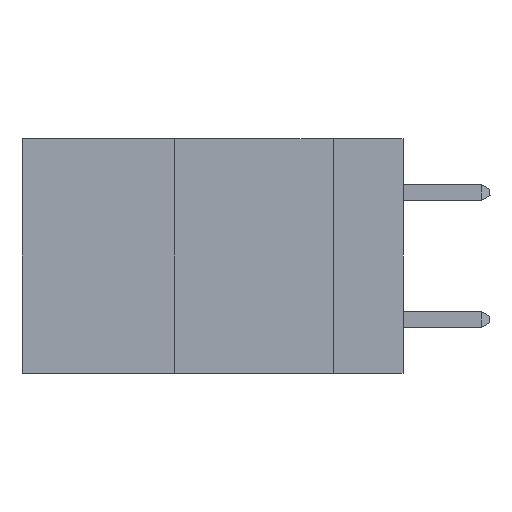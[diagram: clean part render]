
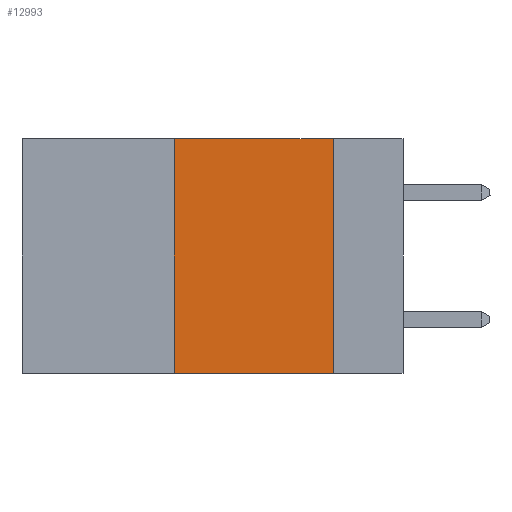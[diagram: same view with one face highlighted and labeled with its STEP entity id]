
A CAD part, left-side view. The second image highlights one B-rep face of the part: STEP entity #12993.
In plain terms, the highlighted planar face has unit normal (-1, 0, 0).
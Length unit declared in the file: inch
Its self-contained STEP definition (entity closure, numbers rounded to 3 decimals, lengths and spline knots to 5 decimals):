
#25 = CARTESIAN_POINT ( 'NONE',  ( 0., 0.36, 0. ) ) ;
#50 = CARTESIAN_POINT ( 'NONE',  ( 0., 0.6, 0. ) ) ;
#1262 = EDGE_LOOP ( 'NONE', ( #12535, #13998, #10342, #11023 ) ) ;
#1325 = PLANE ( 'NONE',  #2939 ) ;
#1431 = VECTOR ( 'NONE', #4845, 39.37008 ) ;
#2601 = VERTEX_POINT ( 'NONE', #15422 ) ;
#2939 = AXIS2_PLACEMENT_3D ( 'NONE', #8607, #13567, #4890 ) ;
#3772 = EDGE_CURVE ( 'NONE', #10120, #2601, #12679, .T. ) ;
#4845 = DIRECTION ( 'NONE',  ( 0., -1., 0. ) ) ;
#4890 = DIRECTION ( 'NONE',  ( 0., 0., -1. ) ) ;
#5891 = CARTESIAN_POINT ( 'NONE',  ( 0., 0.11, 0. ) ) ;
#6127 = VECTOR ( 'NONE', #9921, 39.37008 ) ;
#6905 = VECTOR ( 'NONE', #9473, 39.37008 ) ;
#8069 = VECTOR ( 'NONE', #13212, 39.37008 ) ;
#8261 = CARTESIAN_POINT ( 'NONE',  ( 0., 0.6, -0.37 ) ) ;
#8562 = CARTESIAN_POINT ( 'NONE',  ( 0., 0.11, 0. ) ) ;
#8607 = CARTESIAN_POINT ( 'NONE',  ( 0., 0.6, 0. ) ) ;
#8717 = LINE ( 'NONE', #50, #1431 ) ;
#9239 = EDGE_CURVE ( 'NONE', #10120, #11282, #14430, .T. ) ;
#9358 = VERTEX_POINT ( 'NONE', #8562 ) ;
#9473 = DIRECTION ( 'NONE',  ( 0., 0., -1. ) ) ;
#9921 = DIRECTION ( 'NONE',  ( 0., 0., 1. ) ) ;
#10120 = VERTEX_POINT ( 'NONE', #13987 ) ;
#10342 = ORIENTED_EDGE ( 'NONE', *, *, #3772, .F. ) ;
#11023 = ORIENTED_EDGE ( 'NONE', *, *, #9239, .T. ) ;
#11087 = EDGE_CURVE ( 'NONE', #9358, #11282, #15532, .T. ) ;
#11145 = CARTESIAN_POINT ( 'NONE',  ( 0., 0.11, -0.37 ) ) ;
#11282 = VERTEX_POINT ( 'NONE', #11145 ) ;
#12438 = FACE_OUTER_BOUND ( 'NONE', #1262, .T. ) ;
#12535 = ORIENTED_EDGE ( 'NONE', *, *, #11087, .F. ) ;
#12679 = LINE ( 'NONE', #25, #6127 ) ;
#12993 = ADVANCED_FACE ( 'NONE', ( #12438 ), #1325, .F. ) ;
#13212 = DIRECTION ( 'NONE',  ( 0., -1., 0. ) ) ;
#13567 = DIRECTION ( 'NONE',  ( 1., 0., 0. ) ) ;
#13987 = CARTESIAN_POINT ( 'NONE',  ( 0., 0.36, -0.37 ) ) ;
#13998 = ORIENTED_EDGE ( 'NONE', *, *, #15261, .F. ) ;
#14430 = LINE ( 'NONE', #8261, #8069 ) ;
#15261 = EDGE_CURVE ( 'NONE', #2601, #9358, #8717, .T. ) ;
#15422 = CARTESIAN_POINT ( 'NONE',  ( 0., 0.36, 0. ) ) ;
#15532 = LINE ( 'NONE', #5891, #6905 ) ;
